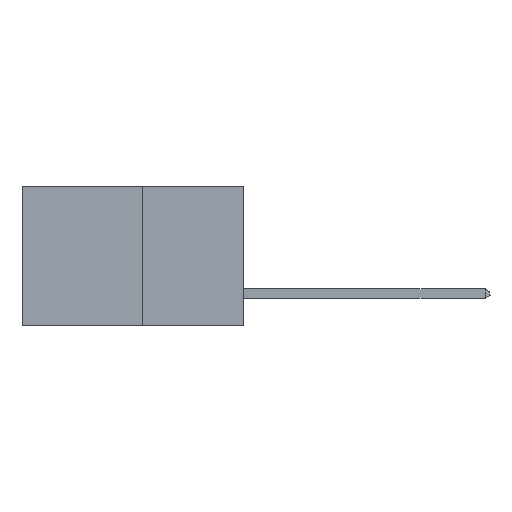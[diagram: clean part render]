
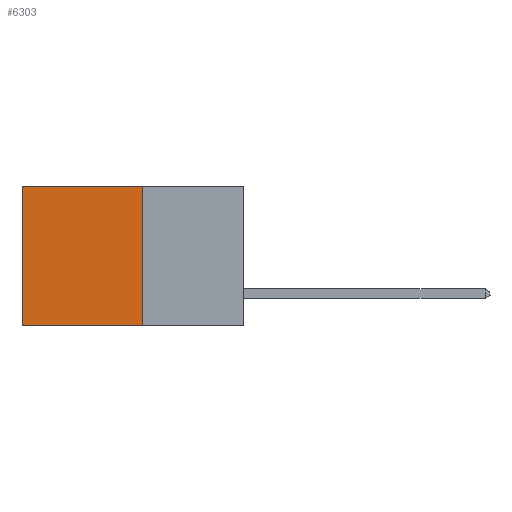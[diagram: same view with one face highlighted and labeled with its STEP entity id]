
A CAD part, left-side view. The second image highlights one B-rep face of the part: STEP entity #6303.
In plain terms, the highlighted planar face has unit normal (-1, 0, 0).
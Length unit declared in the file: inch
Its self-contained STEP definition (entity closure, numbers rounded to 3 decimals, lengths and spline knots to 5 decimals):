
#237 = DIRECTION ( 'NONE',  ( 0., 0., -1. ) ) ;
#314 = DIRECTION ( 'NONE',  ( 1., 0., 0. ) ) ;
#430 = CARTESIAN_POINT ( 'NONE',  ( 0.277, 0.27, -0.37 ) ) ;
#644 = PLANE ( 'NONE',  #683 ) ;
#683 = AXIS2_PLACEMENT_3D ( 'NONE', #430, #314, #237 ) ;
#740 = LINE ( 'NONE', #5425, #9758 ) ;
#1649 = VECTOR ( 'NONE', #6478, 39.37008 ) ;
#2546 = VERTEX_POINT ( 'NONE', #18254 ) ;
#3401 = ORIENTED_EDGE ( 'NONE', *, *, #14457, .F. ) ;
#3402 = EDGE_LOOP ( 'NONE', ( #18742, #20353, #3401, #14471 ) ) ;
#3715 = CARTESIAN_POINT ( 'NONE',  ( 0.277, 0.27, 0. ) ) ;
#3844 = DIRECTION ( 'NONE',  ( 0., 0., -1. ) ) ;
#3874 = EDGE_CURVE ( 'NONE', #2546, #10176, #740, .T. ) ;
#4672 = CARTESIAN_POINT ( 'NONE',  ( 0.277, 0.27, -0.37 ) ) ;
#5425 = CARTESIAN_POINT ( 'NONE',  ( 0.277, 0.27, -0.37 ) ) ;
#5809 = DIRECTION ( 'NONE',  ( 0., 1., 0. ) ) ;
#6303 = ADVANCED_FACE ( 'NONE', ( #11123 ), #644, .F. ) ;
#6478 = DIRECTION ( 'NONE',  ( 0., 0., -1. ) ) ;
#7151 = CARTESIAN_POINT ( 'NONE',  ( 0.277, 0.59, -0.37 ) ) ;
#8296 = VERTEX_POINT ( 'NONE', #3715 ) ;
#9294 = EDGE_CURVE ( 'NONE', #8296, #17752, #11531, .T. ) ;
#9506 = LINE ( 'NONE', #14430, #18177 ) ;
#9758 = VECTOR ( 'NONE', #5809, 39.37008 ) ;
#10176 = VERTEX_POINT ( 'NONE', #7151 ) ;
#10412 = CARTESIAN_POINT ( 'NONE',  ( 0.277, 0.59, 0. ) ) ;
#11123 = FACE_OUTER_BOUND ( 'NONE', #3402, .T. ) ;
#11224 = LINE ( 'NONE', #4672, #1649 ) ;
#11531 = LINE ( 'NONE', #17049, #20442 ) ;
#14430 = CARTESIAN_POINT ( 'NONE',  ( 0.277, 0.59, -0.37 ) ) ;
#14457 = EDGE_CURVE ( 'NONE', #8296, #2546, #11224, .T. ) ;
#14471 = ORIENTED_EDGE ( 'NONE', *, *, #9294, .T. ) ;
#15776 = EDGE_CURVE ( 'NONE', #17752, #10176, #9506, .T. ) ;
#17049 = CARTESIAN_POINT ( 'NONE',  ( 0.277, 0.27, 0. ) ) ;
#17752 = VERTEX_POINT ( 'NONE', #10412 ) ;
#18177 = VECTOR ( 'NONE', #3844, 39.37008 ) ;
#18254 = CARTESIAN_POINT ( 'NONE',  ( 0.277, 0.27, -0.37 ) ) ;
#18742 = ORIENTED_EDGE ( 'NONE', *, *, #15776, .T. ) ;
#18769 = DIRECTION ( 'NONE',  ( 0., 1., 0. ) ) ;
#20353 = ORIENTED_EDGE ( 'NONE', *, *, #3874, .F. ) ;
#20442 = VECTOR ( 'NONE', #18769, 39.37008 ) ;
